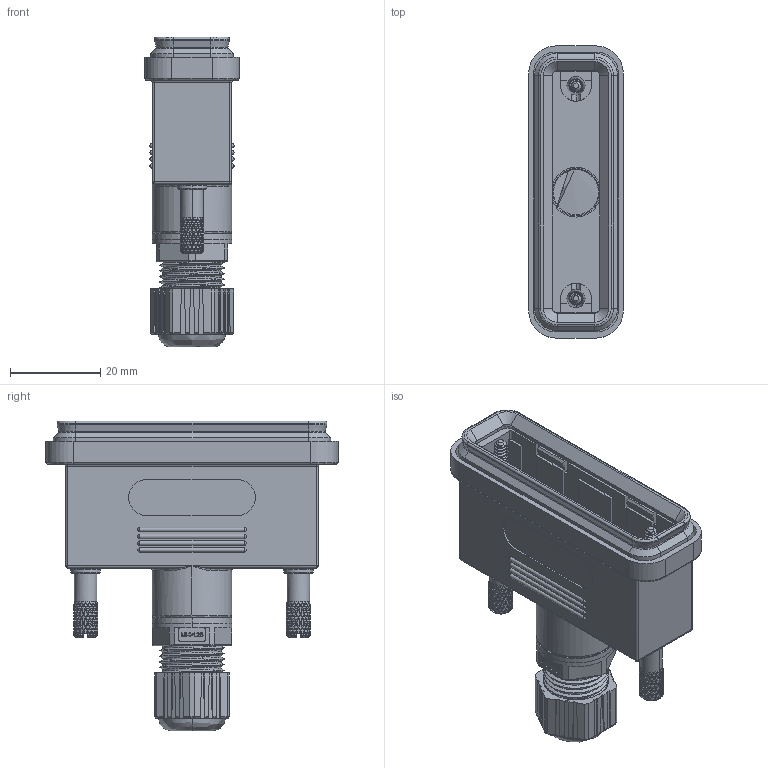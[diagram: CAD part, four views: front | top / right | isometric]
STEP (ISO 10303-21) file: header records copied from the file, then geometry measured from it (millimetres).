
FILE_DESCRIPTION (( 'STEP AP214' ), '1' );
FILE_NAME ('627-230-025-010.STEP', '2020-09-16T21:07:27', ( '' ), ( '' ), 'SwSTEP 2.0', 'SolidWorks 2020', '' );
FILE_SCHEMA (( 'AUTOMOTIVE_DESIGN' ));
Length unit declared in the file: millimetre
Products named in the file (9): O-Ring S; Clamp Nut; Main Body 25; Seal 25; Cable Seal; 627-230-025-010; Cable Guide; O-Ring L; Thumbsrcew
Assembly tree (10 placements, depth 2):
  627-230-025-010
    Main Body 25
    O-Ring S  x2
    Thumbsrcew  x2
    O-Ring L
    Cable Guide
    Cable Seal
    Clamp Nut
    Seal 25
Bounding box: 20.9 x 64.59 x 68.5 mm (x, y, z)
Volume: 6743 mm3; surface area: 22745.2 mm2
Topology: 9 solids, 10 shells, 2767 faces, 6370 edges, 3647 vertices
Faces by surface type: bspline 1559, plane 541, cylinder 539, cone 118, torus 10
Entity records: 88883 total; most frequent: CARTESIAN_POINT 54062, ORIENTED_EDGE 8680, DIRECTION 4404, EDGE_CURVE 4341, VERTEX_POINT 2573, B_SPLINE_CURVE_WITH_KNOTS 2307, EDGE_LOOP 1863, ADVANCED_FACE 1814
